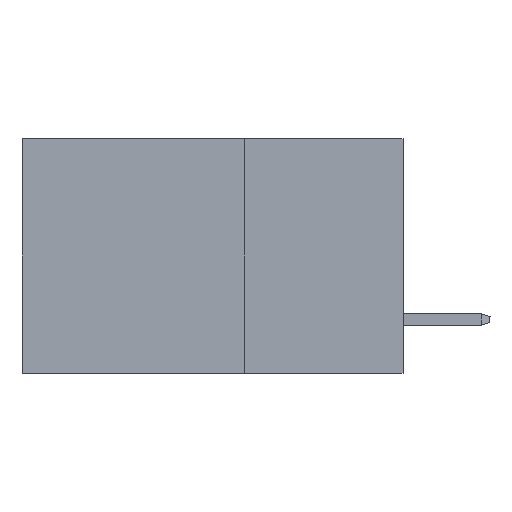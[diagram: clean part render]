
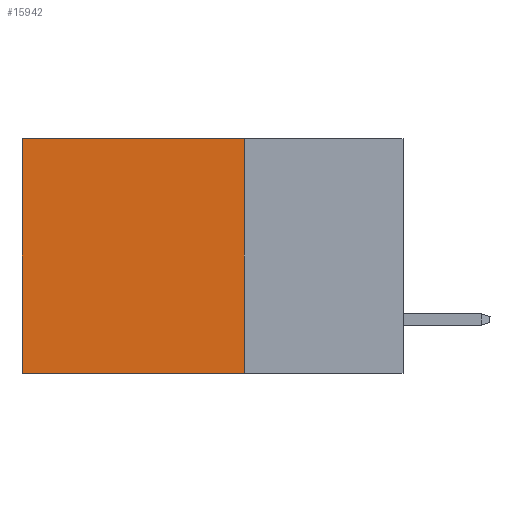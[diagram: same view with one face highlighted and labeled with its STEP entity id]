
A CAD part, left-side view. The second image highlights one B-rep face of the part: STEP entity #15942.
In plain terms, the highlighted planar face has unit normal (-1, 0, 0).
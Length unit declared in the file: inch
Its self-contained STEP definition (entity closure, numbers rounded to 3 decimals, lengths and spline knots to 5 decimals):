
#622 = EDGE_CURVE ( 'NONE', #16102, #28655, #29628, .T. ) ;
#1311 = CARTESIAN_POINT ( 'NONE',  ( 0.2875, 0.6, 0. ) ) ;
#4263 = CARTESIAN_POINT ( 'NONE',  ( 0.2875, 0.25, -0.37 ) ) ;
#7375 = LINE ( 'NONE', #4263, #8732 ) ;
#7888 = VERTEX_POINT ( 'NONE', #37483 ) ;
#8732 = VECTOR ( 'NONE', #22570, 39.37008 ) ;
#10037 = VECTOR ( 'NONE', #11762, 39.37008 ) ;
#10558 = DIRECTION ( 'NONE',  ( 1., 0., 0. ) ) ;
#10882 = EDGE_CURVE ( 'NONE', #26282, #7888, #7375, .T. ) ;
#10960 = CARTESIAN_POINT ( 'NONE',  ( 0.2875, 0.25, 0. ) ) ;
#11762 = DIRECTION ( 'NONE',  ( 0., 1., 0. ) ) ;
#12827 = EDGE_CURVE ( 'NONE', #16102, #26282, #14043, .T. ) ;
#14043 = LINE ( 'NONE', #14233, #27502 ) ;
#14233 = CARTESIAN_POINT ( 'NONE',  ( 0.2875, 0.25, 0. ) ) ;
#15942 = ADVANCED_FACE ( 'NONE', ( #23032 ), #37390, .F. ) ;
#16102 = VERTEX_POINT ( 'NONE', #20507 ) ;
#16964 = LINE ( 'NONE', #19488, #33966 ) ;
#17375 = ORIENTED_EDGE ( 'NONE', *, *, #20600, .T. ) ;
#19488 = CARTESIAN_POINT ( 'NONE',  ( 0.2875, 0.6, 0. ) ) ;
#20507 = CARTESIAN_POINT ( 'NONE',  ( 0.2875, 0.25, 0. ) ) ;
#20600 = EDGE_CURVE ( 'NONE', #28655, #7888, #16964, .T. ) ;
#21074 = CARTESIAN_POINT ( 'NONE',  ( 0.2875, 0.25, 0. ) ) ;
#22432 = CARTESIAN_POINT ( 'NONE',  ( 0.2875, 0.25, -0.37 ) ) ;
#22570 = DIRECTION ( 'NONE',  ( 0., 1., 0. ) ) ;
#23032 = FACE_OUTER_BOUND ( 'NONE', #34910, .T. ) ;
#26282 = VERTEX_POINT ( 'NONE', #22432 ) ;
#27502 = VECTOR ( 'NONE', #31911, 39.37008 ) ;
#28655 = VERTEX_POINT ( 'NONE', #1311 ) ;
#29628 = LINE ( 'NONE', #21074, #10037 ) ;
#30419 = ORIENTED_EDGE ( 'NONE', *, *, #622, .T. ) ;
#31911 = DIRECTION ( 'NONE',  ( 0., 0., -1. ) ) ;
#31935 = AXIS2_PLACEMENT_3D ( 'NONE', #10960, #10558, #34717 ) ;
#32083 = ORIENTED_EDGE ( 'NONE', *, *, #12827, .F. ) ;
#33966 = VECTOR ( 'NONE', #37732, 39.37008 ) ;
#34485 = ORIENTED_EDGE ( 'NONE', *, *, #10882, .F. ) ;
#34717 = DIRECTION ( 'NONE',  ( 0., 0., -1. ) ) ;
#34910 = EDGE_LOOP ( 'NONE', ( #17375, #34485, #32083, #30419 ) ) ;
#37390 = PLANE ( 'NONE',  #31935 ) ;
#37483 = CARTESIAN_POINT ( 'NONE',  ( 0.2875, 0.6, -0.37 ) ) ;
#37732 = DIRECTION ( 'NONE',  ( 0., 0., -1. ) ) ;
